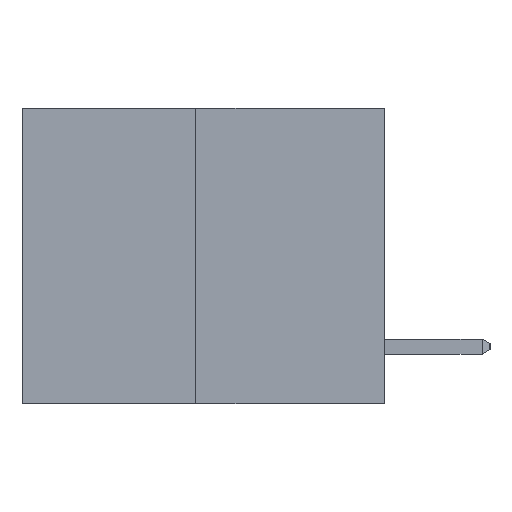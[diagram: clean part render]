
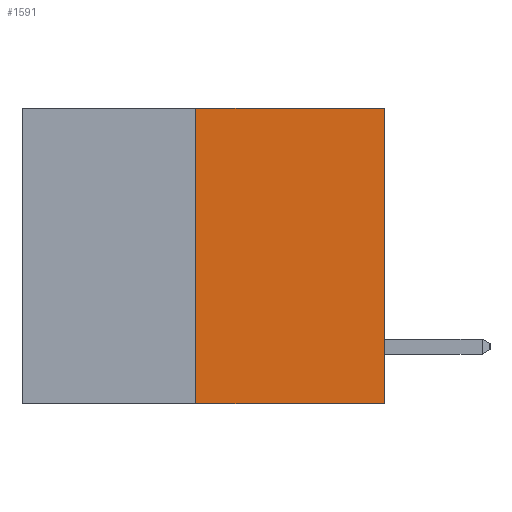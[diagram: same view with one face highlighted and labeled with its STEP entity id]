
A CAD part, left-side view. The second image highlights one B-rep face of the part: STEP entity #1591.
In plain terms, the highlighted planar face has unit normal (-1, 0, 0).
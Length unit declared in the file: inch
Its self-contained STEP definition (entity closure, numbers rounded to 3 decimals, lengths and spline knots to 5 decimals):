
#434 = FACE_OUTER_BOUND ( 'NONE', #9108, .T. ) ;
#482 = EDGE_CURVE ( 'NONE', #3175, #2729, #1432, .T. ) ;
#635 = DIRECTION ( 'NONE',  ( 0., -1., 0. ) ) ;
#872 = CARTESIAN_POINT ( 'NONE',  ( 0., 0.6, -0.49 ) ) ;
#1065 = ORIENTED_EDGE ( 'NONE', *, *, #1461, .F. ) ;
#1172 = LINE ( 'NONE', #1196, #9266 ) ;
#1196 = CARTESIAN_POINT ( 'NONE',  ( 0., 0.312, -0.49 ) ) ;
#1432 = LINE ( 'NONE', #3874, #3764 ) ;
#1461 = EDGE_CURVE ( 'NONE', #3043, #3175, #1172, .T. ) ;
#1591 = ADVANCED_FACE ( 'NONE', ( #434 ), #2770, .F. ) ;
#2078 = DIRECTION ( 'NONE',  ( 0., 0., 1. ) ) ;
#2186 = DIRECTION ( 'NONE',  ( 0., 0., 1. ) ) ;
#2320 = EDGE_CURVE ( 'NONE', #3043, #4466, #3829, .T. ) ;
#2585 = LINE ( 'NONE', #5215, #6105 ) ;
#2729 = VERTEX_POINT ( 'NONE', #5905 ) ;
#2770 = PLANE ( 'NONE',  #7266 ) ;
#2802 = CARTESIAN_POINT ( 'NONE',  ( 0., 0.6, 0. ) ) ;
#3043 = VERTEX_POINT ( 'NONE', #4721 ) ;
#3175 = VERTEX_POINT ( 'NONE', #4081 ) ;
#3309 = EDGE_CURVE ( 'NONE', #4466, #2729, #2585, .T. ) ;
#3600 = DIRECTION ( 'NONE',  ( 1., 0., 0. ) ) ;
#3634 = DIRECTION ( 'NONE',  ( 0., 0., -1. ) ) ;
#3764 = VECTOR ( 'NONE', #635, 39.37008 ) ;
#3829 = LINE ( 'NONE', #872, #6132 ) ;
#3874 = CARTESIAN_POINT ( 'NONE',  ( 0., 0.6, 0. ) ) ;
#3945 = DIRECTION ( 'NONE',  ( 0., -1., 0. ) ) ;
#4081 = CARTESIAN_POINT ( 'NONE',  ( 0., 0.312, 0. ) ) ;
#4466 = VERTEX_POINT ( 'NONE', #4729 ) ;
#4721 = CARTESIAN_POINT ( 'NONE',  ( 0., 0.312, -0.49 ) ) ;
#4729 = CARTESIAN_POINT ( 'NONE',  ( 0., 0., -0.49 ) ) ;
#5215 = CARTESIAN_POINT ( 'NONE',  ( 0., 0., 0. ) ) ;
#5905 = CARTESIAN_POINT ( 'NONE',  ( 0., 0., 0. ) ) ;
#6017 = ORIENTED_EDGE ( 'NONE', *, *, #482, .F. ) ;
#6105 = VECTOR ( 'NONE', #2186, 39.37008 ) ;
#6132 = VECTOR ( 'NONE', #3945, 39.37008 ) ;
#6707 = ORIENTED_EDGE ( 'NONE', *, *, #2320, .T. ) ;
#7266 = AXIS2_PLACEMENT_3D ( 'NONE', #2802, #3600, #3634 ) ;
#9108 = EDGE_LOOP ( 'NONE', ( #1065, #6707, #9783, #6017 ) ) ;
#9266 = VECTOR ( 'NONE', #2078, 39.37008 ) ;
#9783 = ORIENTED_EDGE ( 'NONE', *, *, #3309, .T. ) ;
